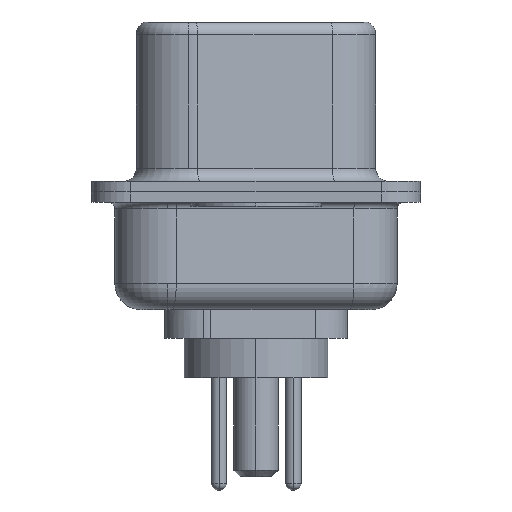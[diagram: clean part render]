
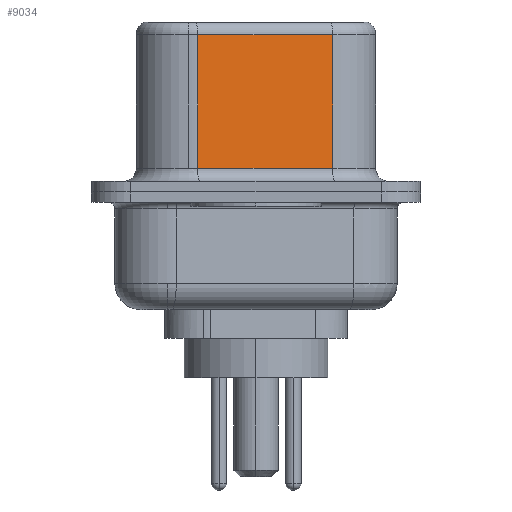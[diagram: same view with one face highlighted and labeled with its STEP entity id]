
A CAD part, left-side view. The second image highlights one B-rep face of the part: STEP entity #9034.
In plain terms, the highlighted planar face has unit normal (-0.985, -0.174, 0).
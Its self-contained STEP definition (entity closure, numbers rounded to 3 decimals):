
#21 = ORIENTED_EDGE ( 'NONE', *, *, #1527, .F. ) ;
#30 = EDGE_CURVE ( 'NONE', #5955, #4996, #6116, .T. ) ;
#834 = DIRECTION ( 'NONE',  ( 0.985, 0.174, 0. ) ) ;
#1527 = EDGE_CURVE ( 'NONE', #10156, #2135, #12665, .T. ) ;
#1546 = EDGE_CURVE ( 'NONE', #4996, #2135, #4491, .T. ) ;
#1696 = ORIENTED_EDGE ( 'NONE', *, *, #1546, .T. ) ;
#1878 = CARTESIAN_POINT ( 'NONE',  ( 4.565, -2.927, 6.52 ) ) ;
#1994 = CARTESIAN_POINT ( 'NONE',  ( 4.565, -2.927, 6.52 ) ) ;
#2057 = ORIENTED_EDGE ( 'NONE', *, *, #30, .T. ) ;
#2135 = VERTEX_POINT ( 'NONE', #5918 ) ;
#3077 = VECTOR ( 'NONE', #11047, 1000. ) ;
#3323 = CARTESIAN_POINT ( 'NONE',  ( 4.565, -2.927, 6.02 ) ) ;
#3390 = VECTOR ( 'NONE', #6695, 1000. ) ;
#4127 = VECTOR ( 'NONE', #7337, 1000. ) ;
#4491 = LINE ( 'NONE', #5614, #4127 ) ;
#4871 = DIRECTION ( 'NONE',  ( 0., 0., -1. ) ) ;
#4996 = VERTEX_POINT ( 'NONE', #12331 ) ;
#5614 = CARTESIAN_POINT ( 'NONE',  ( 4.565, -2.927, 0.9 ) ) ;
#5918 = CARTESIAN_POINT ( 'NONE',  ( 4.565, -2.927, 0.9 ) ) ;
#5955 = VERTEX_POINT ( 'NONE', #11434 ) ;
#6108 = AXIS2_PLACEMENT_3D ( 'NONE', #1994, #834, #11630 ) ;
#6116 = LINE ( 'NONE', #6945, #3077 ) ;
#6378 = LINE ( 'NONE', #3323, #3390 ) ;
#6577 = FACE_OUTER_BOUND ( 'NONE', #10601, .T. ) ;
#6695 = DIRECTION ( 'NONE',  ( -0.174, 0.985, 0. ) ) ;
#6945 = CARTESIAN_POINT ( 'NONE',  ( 3.655, 2.233, 6.52 ) ) ;
#7337 = DIRECTION ( 'NONE',  ( 0.174, -0.985, 0. ) ) ;
#9034 = ADVANCED_FACE ( 'NONE', ( #6577 ), #10677, .F. ) ;
#9828 = VECTOR ( 'NONE', #4871, 1000. ) ;
#10156 = VERTEX_POINT ( 'NONE', #11279 ) ;
#10475 = EDGE_CURVE ( 'NONE', #10156, #5955, #6378, .T. ) ;
#10601 = EDGE_LOOP ( 'NONE', ( #21, #13225, #2057, #1696 ) ) ;
#10677 = PLANE ( 'NONE',  #6108 ) ;
#11047 = DIRECTION ( 'NONE',  ( 0., 0., -1. ) ) ;
#11279 = CARTESIAN_POINT ( 'NONE',  ( 4.565, -2.927, 6.02 ) ) ;
#11434 = CARTESIAN_POINT ( 'NONE',  ( 3.655, 2.233, 6.02 ) ) ;
#11630 = DIRECTION ( 'NONE',  ( -0.174, 0.985, 0. ) ) ;
#12331 = CARTESIAN_POINT ( 'NONE',  ( 3.655, 2.233, 0.9 ) ) ;
#12665 = LINE ( 'NONE', #1878, #9828 ) ;
#13225 = ORIENTED_EDGE ( 'NONE', *, *, #10475, .T. ) ;
